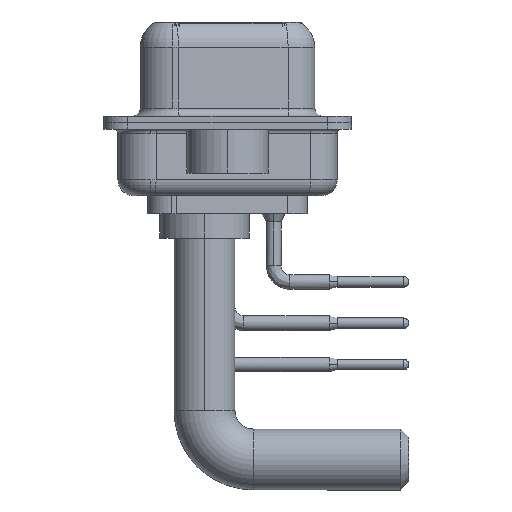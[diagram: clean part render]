
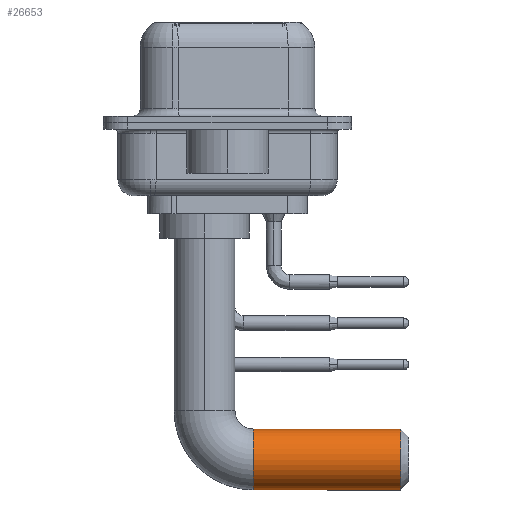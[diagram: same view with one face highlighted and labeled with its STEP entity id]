
A CAD part, left-side view. The second image highlights one B-rep face of the part: STEP entity #26653.
In plain terms, the highlighted cylindrical face has radius 1.875 mm (diameter 3.75 mm), a partial arc.
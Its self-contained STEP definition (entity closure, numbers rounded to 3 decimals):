
#650 = VECTOR ( 'NONE', #28237, 1000. ) ;
#1616 = DIRECTION ( 'NONE',  ( 0., 0., -1. ) ) ;
#2350 = DIRECTION ( 'NONE',  ( -1., 0., 0. ) ) ;
#4296 = CARTESIAN_POINT ( 'NONE',  ( 0., -3., -15.505 ) ) ;
#5404 = LINE ( 'NONE', #4296, #17649 ) ;
#5935 = VERTEX_POINT ( 'NONE', #30415 ) ;
#6427 = AXIS2_PLACEMENT_3D ( 'NONE', #24937, #19677, #2350 ) ;
#8911 = ORIENTED_EDGE ( 'NONE', *, *, #25959, .F. ) ;
#13203 = CARTESIAN_POINT ( 'NONE',  ( 0., -12.07, -13.63 ) ) ;
#13685 = VERTEX_POINT ( 'NONE', #32487 ) ;
#13802 = ORIENTED_EDGE ( 'NONE', *, *, #27935, .T. ) ;
#13930 = CIRCLE ( 'NONE', #32372, 1.875 ) ;
#14053 = EDGE_LOOP ( 'NONE', ( #8911, #21560, #31104, #13802 ) ) ;
#16283 = CARTESIAN_POINT ( 'NONE',  ( 0., -3., -13.63 ) ) ;
#16956 = CYLINDRICAL_SURFACE ( 'NONE', #24382, 1.875 ) ;
#17209 = VERTEX_POINT ( 'NONE', #17256 ) ;
#17256 = CARTESIAN_POINT ( 'NONE',  ( 0., -12.07, -15.505 ) ) ;
#17649 = VECTOR ( 'NONE', #19296, 1000. ) ;
#17688 = DIRECTION ( 'NONE',  ( 0., 1., 0. ) ) ;
#17844 = DIRECTION ( 'NONE',  ( 0., 0., -1. ) ) ;
#19296 = DIRECTION ( 'NONE',  ( 0., -1., 0. ) ) ;
#19586 = CIRCLE ( 'NONE', #6427, 1.875 ) ;
#19677 = DIRECTION ( 'NONE',  ( 0., -1., 0. ) ) ;
#20501 = LINE ( 'NONE', #25292, #650 ) ;
#21560 = ORIENTED_EDGE ( 'NONE', *, *, #24077, .T. ) ;
#24077 = EDGE_CURVE ( 'NONE', #13685, #5935, #19586, .T. ) ;
#24382 = AXIS2_PLACEMENT_3D ( 'NONE', #16283, #26996, #1616 ) ;
#24937 = CARTESIAN_POINT ( 'NONE',  ( 0., -3., -13.63 ) ) ;
#25292 = CARTESIAN_POINT ( 'NONE',  ( 0., -3., -11.755 ) ) ;
#25959 = EDGE_CURVE ( 'NONE', #13685, #28326, #20501, .T. ) ;
#26653 = ADVANCED_FACE ( 'NONE', ( #26658 ), #16956, .T. ) ;
#26658 = FACE_OUTER_BOUND ( 'NONE', #14053, .T. ) ;
#26996 = DIRECTION ( 'NONE',  ( 0., -1., 0. ) ) ;
#27935 = EDGE_CURVE ( 'NONE', #17209, #28326, #13930, .T. ) ;
#28220 = EDGE_CURVE ( 'NONE', #5935, #17209, #5404, .T. ) ;
#28237 = DIRECTION ( 'NONE',  ( 0., -1., 0. ) ) ;
#28326 = VERTEX_POINT ( 'NONE', #32320 ) ;
#30415 = CARTESIAN_POINT ( 'NONE',  ( 0., -3., -15.505 ) ) ;
#31104 = ORIENTED_EDGE ( 'NONE', *, *, #28220, .T. ) ;
#32320 = CARTESIAN_POINT ( 'NONE',  ( 0., -12.07, -11.755 ) ) ;
#32372 = AXIS2_PLACEMENT_3D ( 'NONE', #13203, #17688, #17844 ) ;
#32487 = CARTESIAN_POINT ( 'NONE',  ( 0., -3., -11.755 ) ) ;
